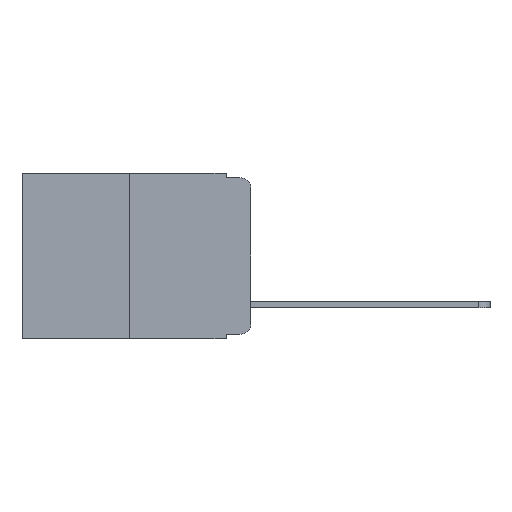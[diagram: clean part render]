
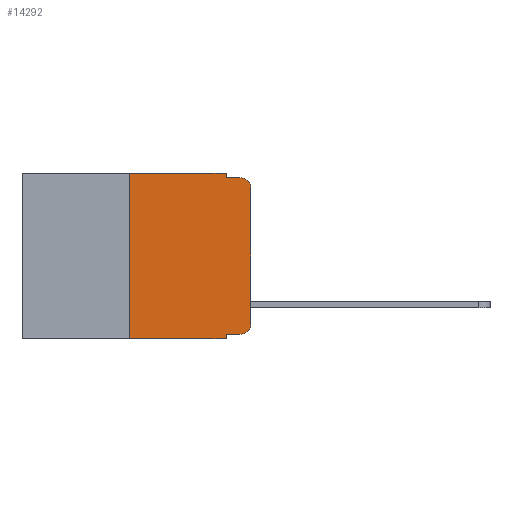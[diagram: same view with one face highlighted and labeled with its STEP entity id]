
A CAD part, left-side view. The second image highlights one B-rep face of the part: STEP entity #14292.
In plain terms, the highlighted planar face has unit normal (-1, 0, 0).
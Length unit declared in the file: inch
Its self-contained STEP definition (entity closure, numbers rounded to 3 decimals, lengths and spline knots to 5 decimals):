
#219 = PLANE ( 'NONE',  #8230 ) ;
#318 = VERTEX_POINT ( 'NONE', #15178 ) ;
#463 = VERTEX_POINT ( 'NONE', #3055 ) ;
#1344 = CARTESIAN_POINT ( 'NONE',  ( 0., 0.25, 0. ) ) ;
#1478 = VECTOR ( 'NONE', #8182, 39.37008 ) ;
#2375 = DIRECTION ( 'NONE',  ( 0., -1., 0. ) ) ;
#2720 = VECTOR ( 'NONE', #10434, 39.37008 ) ;
#2851 = CARTESIAN_POINT ( 'NONE',  ( 0., 0.051, -0.01 ) ) ;
#2983 = CARTESIAN_POINT ( 'NONE',  ( 0., 0.051, 0. ) ) ;
#3055 = CARTESIAN_POINT ( 'NONE',  ( 0., 0.02, -0.333 ) ) ;
#3225 = ORIENTED_EDGE ( 'NONE', *, *, #21044, .T. ) ;
#3238 = DIRECTION ( 'NONE',  ( 0., 0., 1. ) ) ;
#3280 = LINE ( 'NONE', #1344, #21053 ) ;
#3711 = ORIENTED_EDGE ( 'NONE', *, *, #21107, .T. ) ;
#3756 = ORIENTED_EDGE ( 'NONE', *, *, #21177, .F. ) ;
#4075 = ORIENTED_EDGE ( 'NONE', *, *, #21233, .F. ) ;
#4105 = LINE ( 'NONE', #19213, #21827 ) ;
#4119 = LINE ( 'NONE', #6419, #8891 ) ;
#4231 = ORIENTED_EDGE ( 'NONE', *, *, #19086, .F. ) ;
#4296 = CARTESIAN_POINT ( 'NONE',  ( 0., 0.473, 0. ) ) ;
#4328 = VERTEX_POINT ( 'NONE', #17852 ) ;
#4872 = ORIENTED_EDGE ( 'NONE', *, *, #21306, .F. ) ;
#4886 = DIRECTION ( 'NONE',  ( 0., 0., -1. ) ) ;
#5449 = DIRECTION ( 'NONE',  ( 0., -1., 0. ) ) ;
#6028 = ORIENTED_EDGE ( 'NONE', *, *, #20576, .T. ) ;
#6419 = CARTESIAN_POINT ( 'NONE',  ( 0., 0.473, -0.343 ) ) ;
#6590 = CARTESIAN_POINT ( 'NONE',  ( 0., 0., -0.03 ) ) ;
#6613 = ORIENTED_EDGE ( 'NONE', *, *, #21311, .F. ) ;
#6862 = VERTEX_POINT ( 'NONE', #11771 ) ;
#6987 = ORIENTED_EDGE ( 'NONE', *, *, #21434, .T. ) ;
#7200 = AXIS2_PLACEMENT_3D ( 'NONE', #18389, #8033, #19967 ) ;
#7299 = ORIENTED_EDGE ( 'NONE', *, *, #21460, .T. ) ;
#7303 = DIRECTION ( 'NONE',  ( -1., 0., 0. ) ) ;
#7936 = DIRECTION ( 'NONE',  ( 0., 0., -1. ) ) ;
#8025 = CIRCLE ( 'NONE', #7200, 0.02 ) ;
#8033 = DIRECTION ( 'NONE',  ( -1., 0., 0. ) ) ;
#8182 = DIRECTION ( 'NONE',  ( 0., -1., 0. ) ) ;
#8223 = VERTEX_POINT ( 'NONE', #19571 ) ;
#8230 = AXIS2_PLACEMENT_3D ( 'NONE', #4296, #18295, #7936 ) ;
#8577 = LINE ( 'NONE', #8607, #2720 ) ;
#8607 = CARTESIAN_POINT ( 'NONE',  ( 0., 0.051, 0. ) ) ;
#8891 = VECTOR ( 'NONE', #13517, 39.37008 ) ;
#9157 = VECTOR ( 'NONE', #4886, 39.37008 ) ;
#9198 = CARTESIAN_POINT ( 'NONE',  ( 0., 0.25, 0. ) ) ;
#9458 = FACE_OUTER_BOUND ( 'NONE', #14196, .T. ) ;
#9535 = CARTESIAN_POINT ( 'NONE',  ( 0., 0.473, 0. ) ) ;
#10392 = VERTEX_POINT ( 'NONE', #15678 ) ;
#10434 = DIRECTION ( 'NONE',  ( 0., 0., -1. ) ) ;
#11771 = CARTESIAN_POINT ( 'NONE',  ( 0., 0.051, -0.01 ) ) ;
#12105 = VERTEX_POINT ( 'NONE', #2983 ) ;
#13150 = CARTESIAN_POINT ( 'NONE',  ( 0., 0.051, -0.333 ) ) ;
#13517 = DIRECTION ( 'NONE',  ( 0., -1., 0. ) ) ;
#13637 = CARTESIAN_POINT ( 'NONE',  ( 0., 0.051, 0. ) ) ;
#13822 = LINE ( 'NONE', #13637, #9157 ) ;
#14196 = EDGE_LOOP ( 'NONE', ( #3225, #3711, #3756, #4075, #4231, #4872, #6028, #6613, #6987, #7299 ) ) ;
#14292 = ADVANCED_FACE ( 'NONE', ( #9458 ), #219, .F. ) ;
#14332 = LINE ( 'NONE', #16612, #14730 ) ;
#14730 = VECTOR ( 'NONE', #18254, 39.37008 ) ;
#15178 = CARTESIAN_POINT ( 'NONE',  ( 0., 0.02, -0.01 ) ) ;
#15678 = CARTESIAN_POINT ( 'NONE',  ( 0., 0.25, -0.343 ) ) ;
#16266 = VERTEX_POINT ( 'NONE', #13150 ) ;
#16612 = CARTESIAN_POINT ( 'NONE',  ( 0., 0., 0. ) ) ;
#16879 = VERTEX_POINT ( 'NONE', #9198 ) ;
#17658 = VECTOR ( 'NONE', #2375, 39.37008 ) ;
#17762 = CARTESIAN_POINT ( 'NONE',  ( 0., 0.02, -0.313 ) ) ;
#17852 = CARTESIAN_POINT ( 'NONE',  ( 0., 0., -0.313 ) ) ;
#18026 = VERTEX_POINT ( 'NONE', #6590 ) ;
#18254 = DIRECTION ( 'NONE',  ( 0., 0., 1. ) ) ;
#18295 = DIRECTION ( 'NONE',  ( 1., 0., 0. ) ) ;
#18389 = CARTESIAN_POINT ( 'NONE',  ( 0., 0.02, -0.03 ) ) ;
#18801 = AXIS2_PLACEMENT_3D ( 'NONE', #17762, #7303, #19336 ) ;
#19086 = EDGE_CURVE ( 'NONE', #16879, #12105, #21885, .T. ) ;
#19213 = CARTESIAN_POINT ( 'NONE',  ( 0., 0.051, -0.333 ) ) ;
#19336 = DIRECTION ( 'NONE',  ( 0., 0., -1. ) ) ;
#19571 = CARTESIAN_POINT ( 'NONE',  ( 0., 0.051, -0.343 ) ) ;
#19967 = DIRECTION ( 'NONE',  ( 0., 0., -1. ) ) ;
#20031 = LINE ( 'NONE', #2851, #1478 ) ;
#20576 = EDGE_CURVE ( 'NONE', #10392, #8223, #4119, .T. ) ;
#21044 = EDGE_CURVE ( 'NONE', #4328, #18026, #14332, .T. ) ;
#21053 = VECTOR ( 'NONE', #3238, 39.37008 ) ;
#21107 = EDGE_CURVE ( 'NONE', #18026, #318, #8025, .T. ) ;
#21177 = EDGE_CURVE ( 'NONE', #6862, #318, #20031, .T. ) ;
#21233 = EDGE_CURVE ( 'NONE', #12105, #6862, #13822, .T. ) ;
#21306 = EDGE_CURVE ( 'NONE', #10392, #16879, #3280, .T. ) ;
#21311 = EDGE_CURVE ( 'NONE', #16266, #8223, #8577, .T. ) ;
#21312 = CIRCLE ( 'NONE', #18801, 0.02 ) ;
#21434 = EDGE_CURVE ( 'NONE', #16266, #463, #4105, .T. ) ;
#21460 = EDGE_CURVE ( 'NONE', #463, #4328, #21312, .T. ) ;
#21827 = VECTOR ( 'NONE', #5449, 39.37008 ) ;
#21885 = LINE ( 'NONE', #9535, #17658 ) ;
